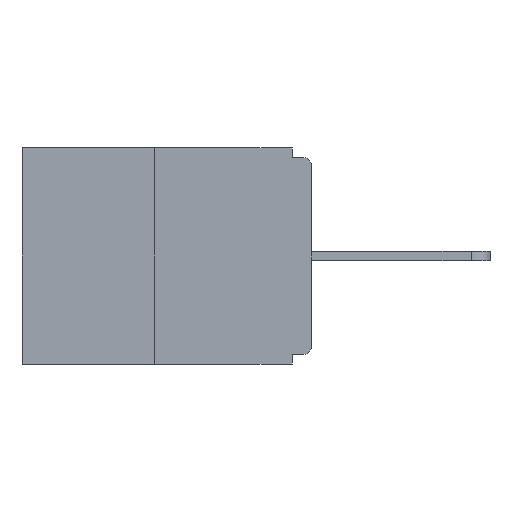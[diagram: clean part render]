
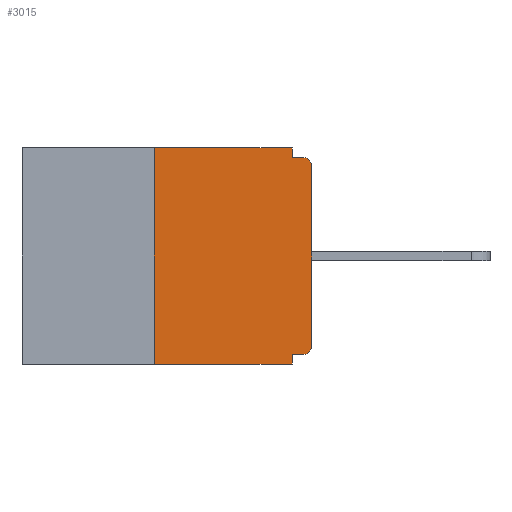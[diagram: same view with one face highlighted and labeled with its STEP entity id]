
A CAD part, left-side view. The second image highlights one B-rep face of the part: STEP entity #3015.
In plain terms, the highlighted planar face has unit normal (-1, 0, 0).
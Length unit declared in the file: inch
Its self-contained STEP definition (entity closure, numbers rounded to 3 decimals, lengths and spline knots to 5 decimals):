
#90 = LINE ( 'NONE', #5386, #3523 ) ;
#487 = AXIS2_PLACEMENT_3D ( 'NONE', #10704, #15291, #15143 ) ;
#695 = CARTESIAN_POINT ( 'NONE',  ( 0., 0.031, 0. ) ) ;
#708 = ORIENTED_EDGE ( 'NONE', *, *, #980, .T. ) ;
#722 = ORIENTED_EDGE ( 'NONE', *, *, #6913, .F. ) ;
#920 = ORIENTED_EDGE ( 'NONE', *, *, #6716, .F. ) ;
#937 = LINE ( 'NONE', #10072, #3941 ) ;
#980 = EDGE_CURVE ( 'NONE', #7156, #5412, #9160, .T. ) ;
#1390 = ORIENTED_EDGE ( 'NONE', *, *, #7503, .T. ) ;
#1682 = ORIENTED_EDGE ( 'NONE', *, *, #8332, .F. ) ;
#1825 = VECTOR ( 'NONE', #4350, 39.37008 ) ;
#2401 = ORIENTED_EDGE ( 'NONE', *, *, #2722, .F. ) ;
#2443 = ORIENTED_EDGE ( 'NONE', *, *, #5887, .F. ) ;
#2538 = VECTOR ( 'NONE', #5066, 39.37008 ) ;
#2722 = EDGE_CURVE ( 'NONE', #3088, #10113, #10325, .T. ) ;
#2806 = ORIENTED_EDGE ( 'NONE', *, *, #7596, .F. ) ;
#2926 = LINE ( 'NONE', #12194, #2538 ) ;
#3010 = CARTESIAN_POINT ( 'NONE',  ( 0., 0., -0.03 ) ) ;
#3015 = ADVANCED_FACE ( 'NONE', ( #12119 ), #7502, .F. ) ;
#3088 = VERTEX_POINT ( 'NONE', #8789 ) ;
#3523 = VECTOR ( 'NONE', #6698, 39.37008 ) ;
#3941 = VECTOR ( 'NONE', #4008, 39.37008 ) ;
#4008 = DIRECTION ( 'NONE',  ( 0., 0., -1. ) ) ;
#4258 = VECTOR ( 'NONE', #14994, 39.37008 ) ;
#4300 = ORIENTED_EDGE ( 'NONE', *, *, #15002, .T. ) ;
#4350 = DIRECTION ( 'NONE',  ( 0., 0., 1. ) ) ;
#4902 = ORIENTED_EDGE ( 'NONE', *, *, #10093, .T. ) ;
#4921 = CARTESIAN_POINT ( 'NONE',  ( 0., 0.015, -0.015 ) ) ;
#5066 = DIRECTION ( 'NONE',  ( 0., 0., -1. ) ) ;
#5386 = CARTESIAN_POINT ( 'NONE',  ( 0., 0., -0.328 ) ) ;
#5412 = VERTEX_POINT ( 'NONE', #11527 ) ;
#5887 = EDGE_CURVE ( 'NONE', #12792, #3088, #937, .T. ) ;
#6069 = VERTEX_POINT ( 'NONE', #3010 ) ;
#6380 = EDGE_LOOP ( 'NONE', ( #2806, #1682, #1390, #920, #722, #708, #4902, #4300, #2401, #2443 ) ) ;
#6520 = CARTESIAN_POINT ( 'NONE',  ( 0., 0.46, -0.343 ) ) ;
#6698 = DIRECTION ( 'NONE',  ( 0., 1., 0. ) ) ;
#6716 = EDGE_CURVE ( 'NONE', #6898, #13044, #2926, .T. ) ;
#6898 = VERTEX_POINT ( 'NONE', #7854 ) ;
#6913 = EDGE_CURVE ( 'NONE', #7156, #6898, #90, .T. ) ;
#7156 = VERTEX_POINT ( 'NONE', #11841 ) ;
#7335 = DIRECTION ( 'NONE',  ( 0., 0., 1. ) ) ;
#7382 = VECTOR ( 'NONE', #8960, 39.37008 ) ;
#7454 = DIRECTION ( 'NONE',  ( -1., 0., 0. ) ) ;
#7460 = CARTESIAN_POINT ( 'NONE',  ( 0., 0.031, -0.343 ) ) ;
#7502 = PLANE ( 'NONE',  #487 ) ;
#7503 = EDGE_CURVE ( 'NONE', #14091, #13044, #10545, .T. ) ;
#7596 = EDGE_CURVE ( 'NONE', #10033, #12792, #9789, .T. ) ;
#7673 = LINE ( 'NONE', #12702, #1825 ) ;
#7765 = AXIS2_PLACEMENT_3D ( 'NONE', #14420, #7454, #15560 ) ;
#7854 = CARTESIAN_POINT ( 'NONE',  ( 0., 0.031, -0.328 ) ) ;
#8332 = EDGE_CURVE ( 'NONE', #14091, #10033, #7673, .T. ) ;
#8405 = CARTESIAN_POINT ( 'NONE',  ( 0., 0.25, 0. ) ) ;
#8567 = LINE ( 'NONE', #14320, #12385 ) ;
#8789 = CARTESIAN_POINT ( 'NONE',  ( 0., 0.031, -0.015 ) ) ;
#8960 = DIRECTION ( 'NONE',  ( 0., -1., 0. ) ) ;
#9160 = CIRCLE ( 'NONE', #11493, 0.015 ) ;
#9349 = CARTESIAN_POINT ( 'NONE',  ( 0., 0.25, -0.343 ) ) ;
#9789 = LINE ( 'NONE', #10300, #12510 ) ;
#10033 = VERTEX_POINT ( 'NONE', #8405 ) ;
#10072 = CARTESIAN_POINT ( 'NONE',  ( 0., 0.031, 0. ) ) ;
#10093 = EDGE_CURVE ( 'NONE', #5412, #6069, #8567, .T. ) ;
#10113 = VERTEX_POINT ( 'NONE', #4921 ) ;
#10300 = CARTESIAN_POINT ( 'NONE',  ( 0., 0.46, 0. ) ) ;
#10325 = LINE ( 'NONE', #11471, #4258 ) ;
#10545 = LINE ( 'NONE', #6520, #7382 ) ;
#10704 = CARTESIAN_POINT ( 'NONE',  ( 0., 0.46, 0. ) ) ;
#11267 = CARTESIAN_POINT ( 'NONE',  ( 0., 0.015, -0.313 ) ) ;
#11390 = DIRECTION ( 'NONE',  ( -1., 0., 0. ) ) ;
#11471 = CARTESIAN_POINT ( 'NONE',  ( 0., 0., -0.015 ) ) ;
#11480 = DIRECTION ( 'NONE',  ( 0., -1., 0. ) ) ;
#11493 = AXIS2_PLACEMENT_3D ( 'NONE', #11267, #11390, #12090 ) ;
#11527 = CARTESIAN_POINT ( 'NONE',  ( 0., 0., -0.313 ) ) ;
#11661 = CIRCLE ( 'NONE', #7765, 0.015 ) ;
#11841 = CARTESIAN_POINT ( 'NONE',  ( 0., 0.015, -0.328 ) ) ;
#12090 = DIRECTION ( 'NONE',  ( 0., 0., -1. ) ) ;
#12119 = FACE_OUTER_BOUND ( 'NONE', #6380, .T. ) ;
#12194 = CARTESIAN_POINT ( 'NONE',  ( 0., 0.031, -0.343 ) ) ;
#12385 = VECTOR ( 'NONE', #7335, 39.37008 ) ;
#12510 = VECTOR ( 'NONE', #11480, 39.37008 ) ;
#12702 = CARTESIAN_POINT ( 'NONE',  ( 0., 0.25, 0. ) ) ;
#12792 = VERTEX_POINT ( 'NONE', #695 ) ;
#13044 = VERTEX_POINT ( 'NONE', #7460 ) ;
#14091 = VERTEX_POINT ( 'NONE', #9349 ) ;
#14320 = CARTESIAN_POINT ( 'NONE',  ( 0., 0., 0. ) ) ;
#14420 = CARTESIAN_POINT ( 'NONE',  ( 0., 0.015, -0.03 ) ) ;
#14994 = DIRECTION ( 'NONE',  ( 0., -1., 0. ) ) ;
#15002 = EDGE_CURVE ( 'NONE', #6069, #10113, #11661, .T. ) ;
#15143 = DIRECTION ( 'NONE',  ( 0., 0., -1. ) ) ;
#15291 = DIRECTION ( 'NONE',  ( 1., 0., 0. ) ) ;
#15560 = DIRECTION ( 'NONE',  ( 0., 0., -1. ) ) ;
